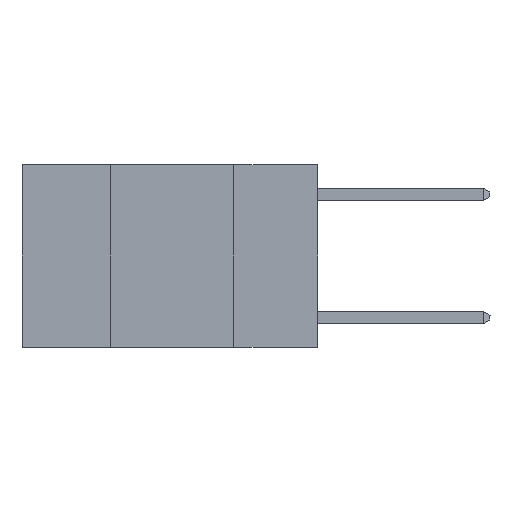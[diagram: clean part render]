
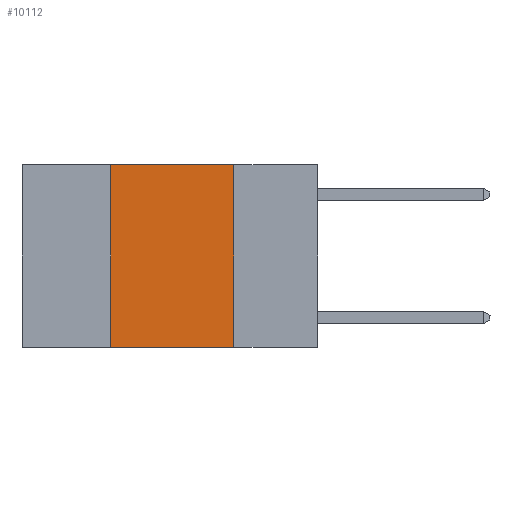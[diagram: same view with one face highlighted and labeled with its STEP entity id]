
A CAD part, left-side view. The second image highlights one B-rep face of the part: STEP entity #10112.
In plain terms, the highlighted planar face has unit normal (-1, 0, 0).
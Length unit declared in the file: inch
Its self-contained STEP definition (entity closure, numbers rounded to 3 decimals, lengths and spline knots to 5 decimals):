
#137 = ORIENTED_EDGE ( 'NONE', *, *, #14826, .F. ) ;
#863 = VECTOR ( 'NONE', #16183, 39.37008 ) ;
#1291 = FACE_OUTER_BOUND ( 'NONE', #22065, .T. ) ;
#1378 = CARTESIAN_POINT ( 'NONE',  ( 0., 0.42, -0.37 ) ) ;
#1814 = CARTESIAN_POINT ( 'NONE',  ( 0., 0.6, 0. ) ) ;
#2725 = CARTESIAN_POINT ( 'NONE',  ( 0., 0.42, 0. ) ) ;
#3665 = DIRECTION ( 'NONE',  ( 0., 0., -1. ) ) ;
#6811 = DIRECTION ( 'NONE',  ( 0., -1., 0. ) ) ;
#7334 = CARTESIAN_POINT ( 'NONE',  ( 0., 0.17, 0. ) ) ;
#7658 = LINE ( 'NONE', #9304, #16464 ) ;
#8346 = CARTESIAN_POINT ( 'NONE',  ( 0., 0.6, 0. ) ) ;
#8452 = VERTEX_POINT ( 'NONE', #1378 ) ;
#9304 = CARTESIAN_POINT ( 'NONE',  ( 0., 0.42, 0. ) ) ;
#9827 = ORIENTED_EDGE ( 'NONE', *, *, #16001, .T. ) ;
#10094 = LINE ( 'NONE', #8346, #14768 ) ;
#10112 = ADVANCED_FACE ( 'NONE', ( #1291 ), #15975, .F. ) ;
#10114 = DIRECTION ( 'NONE',  ( 0., -1., 0. ) ) ;
#10469 = LINE ( 'NONE', #7334, #863 ) ;
#11040 = VERTEX_POINT ( 'NONE', #20006 ) ;
#11084 = DIRECTION ( 'NONE',  ( 0., 0., 1. ) ) ;
#12643 = VERTEX_POINT ( 'NONE', #2725 ) ;
#12941 = CARTESIAN_POINT ( 'NONE',  ( 0., 0.17, -0.37 ) ) ;
#13634 = EDGE_CURVE ( 'NONE', #11040, #13754, #10469, .T. ) ;
#13754 = VERTEX_POINT ( 'NONE', #12941 ) ;
#14276 = DIRECTION ( 'NONE',  ( 1., 0., 0. ) ) ;
#14768 = VECTOR ( 'NONE', #10114, 39.37008 ) ;
#14826 = EDGE_CURVE ( 'NONE', #8452, #12643, #7658, .T. ) ;
#15975 = PLANE ( 'NONE',  #17188 ) ;
#16001 = EDGE_CURVE ( 'NONE', #8452, #13754, #22904, .T. ) ;
#16183 = DIRECTION ( 'NONE',  ( 0., 0., -1. ) ) ;
#16464 = VECTOR ( 'NONE', #11084, 39.37008 ) ;
#17188 = AXIS2_PLACEMENT_3D ( 'NONE', #1814, #14276, #3665 ) ;
#18081 = ORIENTED_EDGE ( 'NONE', *, *, #13634, .F. ) ;
#18281 = VECTOR ( 'NONE', #6811, 39.37008 ) ;
#18635 = ORIENTED_EDGE ( 'NONE', *, *, #20883, .F. ) ;
#20006 = CARTESIAN_POINT ( 'NONE',  ( 0., 0.17, 0. ) ) ;
#20879 = CARTESIAN_POINT ( 'NONE',  ( 0., 0.6, -0.37 ) ) ;
#20883 = EDGE_CURVE ( 'NONE', #12643, #11040, #10094, .T. ) ;
#22065 = EDGE_LOOP ( 'NONE', ( #18081, #18635, #137, #9827 ) ) ;
#22904 = LINE ( 'NONE', #20879, #18281 ) ;
